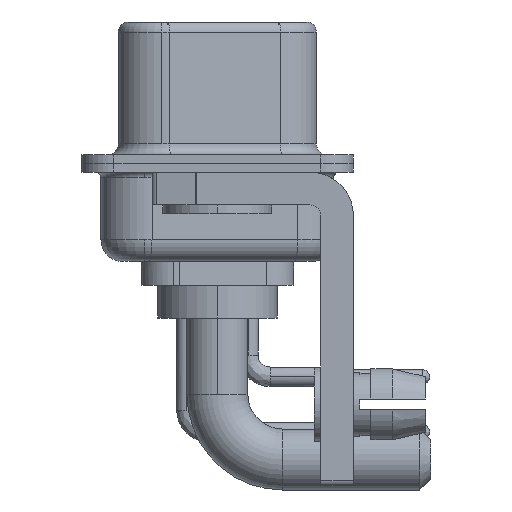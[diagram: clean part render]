
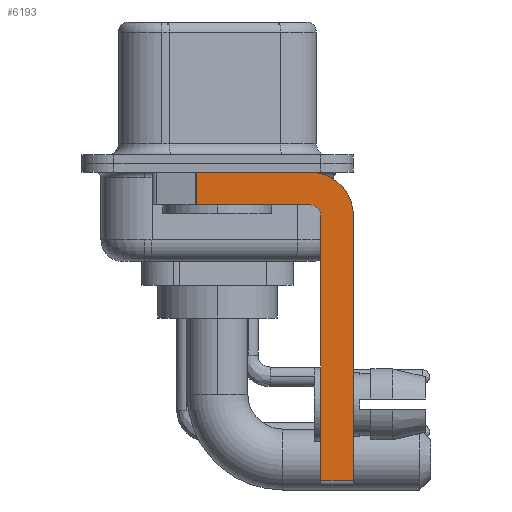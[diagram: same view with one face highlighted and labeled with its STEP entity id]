
A CAD part, left-side view. The second image highlights one B-rep face of the part: STEP entity #6193.
In plain terms, the highlighted planar face has unit normal (-1, 0, 0).
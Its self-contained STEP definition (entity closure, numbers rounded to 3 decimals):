
#279 = ORIENTED_EDGE ( 'NONE', *, *, #3281, .T. ) ;
#308 = ORIENTED_EDGE ( 'NONE', *, *, #6613, .T. ) ;
#580 = VERTEX_POINT ( 'NONE', #21489 ) ;
#977 = DIRECTION ( 'NONE',  ( 0., -1., 0. ) ) ;
#2614 = VERTEX_POINT ( 'NONE', #24230 ) ;
#2747 = VERTEX_POINT ( 'NONE', #26788 ) ;
#2781 = VERTEX_POINT ( 'NONE', #24901 ) ;
#2884 = CARTESIAN_POINT ( 'NONE',  ( -2.9, -4.25, -14.55 ) ) ;
#3281 = EDGE_CURVE ( 'NONE', #2747, #580, #25531, .T. ) ;
#3581 = EDGE_LOOP ( 'NONE', ( #22573, #279, #25792, #25350, #11338, #308, #6812, #4042 ) ) ;
#4042 = ORIENTED_EDGE ( 'NONE', *, *, #8808, .F. ) ;
#4413 = VERTEX_POINT ( 'NONE', #24467 ) ;
#4415 = VERTEX_POINT ( 'NONE', #5698 ) ;
#4446 = CARTESIAN_POINT ( 'NONE',  ( -2.9, -6.25, -2.4 ) ) ;
#4888 = DIRECTION ( 'NONE',  ( 0., 0., -1. ) ) ;
#5067 = VECTOR ( 'NONE', #977, 1000. ) ;
#5698 = CARTESIAN_POINT ( 'NONE',  ( -2.9, -4.75, -14.55 ) ) ;
#6134 = CARTESIAN_POINT ( 'NONE',  ( -2.9, -4.25, -2.4 ) ) ;
#6193 = ADVANCED_FACE ( 'NONE', ( #21496 ), #15644, .F. ) ;
#6613 = EDGE_CURVE ( 'NONE', #4415, #12518, #17320, .T. ) ;
#6812 = ORIENTED_EDGE ( 'NONE', *, *, #21670, .F. ) ;
#6926 = DIRECTION ( 'NONE',  ( 0., 0., -1. ) ) ;
#7374 = DIRECTION ( 'NONE',  ( 0., 0., -1. ) ) ;
#7470 = DIRECTION ( 'NONE',  ( 0., 0., -1. ) ) ;
#7517 = CIRCLE ( 'NONE', #9676, 0.5 ) ;
#8808 = EDGE_CURVE ( 'NONE', #4413, #26354, #25456, .T. ) ;
#8908 = LINE ( 'NONE', #9443, #19947 ) ;
#9243 = EDGE_CURVE ( 'NONE', #2747, #4413, #21679, .T. ) ;
#9312 = AXIS2_PLACEMENT_3D ( 'NONE', #11714, #11445, #4888 ) ;
#9443 = CARTESIAN_POINT ( 'NONE',  ( -2.9, -4.75, -14.8 ) ) ;
#9655 = DIRECTION ( 'NONE',  ( 0., 1., 0. ) ) ;
#9676 = AXIS2_PLACEMENT_3D ( 'NONE', #6134, #18091, #24222 ) ;
#10890 = VECTOR ( 'NONE', #7374, 1000. ) ;
#11122 = CARTESIAN_POINT ( 'NONE',  ( -2.9, 0.978, -1.9 ) ) ;
#11203 = DIRECTION ( 'NONE',  ( 0., -1., 0. ) ) ;
#11338 = ORIENTED_EDGE ( 'NONE', *, *, #20989, .F. ) ;
#11414 = CARTESIAN_POINT ( 'NONE',  ( -2.9, -4.25, -2.4 ) ) ;
#11445 = DIRECTION ( 'NONE',  ( 1., 0., 0. ) ) ;
#11714 = CARTESIAN_POINT ( 'NONE',  ( -2.9, -4.25, -2.4 ) ) ;
#11848 = LINE ( 'NONE', #24344, #10890 ) ;
#12518 = VERTEX_POINT ( 'NONE', #17530 ) ;
#13582 = DIRECTION ( 'NONE',  ( 1., 0., 0. ) ) ;
#13995 = LINE ( 'NONE', #25945, #18720 ) ;
#15644 = PLANE ( 'NONE',  #9312 ) ;
#17320 = LINE ( 'NONE', #2884, #21898 ) ;
#17530 = CARTESIAN_POINT ( 'NONE',  ( -2.9, -6.25, -14.55 ) ) ;
#18091 = DIRECTION ( 'NONE',  ( -1., 0., 0. ) ) ;
#18523 = AXIS2_PLACEMENT_3D ( 'NONE', #11414, #13582, #7470 ) ;
#18720 = VECTOR ( 'NONE', #9655, 1000. ) ;
#19947 = VECTOR ( 'NONE', #25476, 1000. ) ;
#20989 = EDGE_CURVE ( 'NONE', #4415, #2781, #8908, .T. ) ;
#21196 = VECTOR ( 'NONE', #6926, 1000. ) ;
#21489 = CARTESIAN_POINT ( 'NONE',  ( -2.9, 0.978, -1.9 ) ) ;
#21496 = FACE_OUTER_BOUND ( 'NONE', #3581, .T. ) ;
#21670 = EDGE_CURVE ( 'NONE', #26354, #12518, #11848, .T. ) ;
#21679 = LINE ( 'NONE', #26002, #5067 ) ;
#21898 = VECTOR ( 'NONE', #11203, 1000. ) ;
#22573 = ORIENTED_EDGE ( 'NONE', *, *, #9243, .F. ) ;
#24222 = DIRECTION ( 'NONE',  ( 0., 0., 1. ) ) ;
#24230 = CARTESIAN_POINT ( 'NONE',  ( -2.9, -4.25, -1.9 ) ) ;
#24344 = CARTESIAN_POINT ( 'NONE',  ( -2.9, -6.25, -2.4 ) ) ;
#24358 = EDGE_CURVE ( 'NONE', #2614, #580, #13995, .T. ) ;
#24467 = CARTESIAN_POINT ( 'NONE',  ( -2.9, -4.25, -0.4 ) ) ;
#24901 = CARTESIAN_POINT ( 'NONE',  ( -2.9, -4.75, -2.4 ) ) ;
#25350 = ORIENTED_EDGE ( 'NONE', *, *, #25757, .F. ) ;
#25456 = CIRCLE ( 'NONE', #18523, 2. ) ;
#25476 = DIRECTION ( 'NONE',  ( 0., 0., 1. ) ) ;
#25531 = LINE ( 'NONE', #11122, #21196 ) ;
#25757 = EDGE_CURVE ( 'NONE', #2781, #2614, #7517, .T. ) ;
#25792 = ORIENTED_EDGE ( 'NONE', *, *, #24358, .F. ) ;
#25945 = CARTESIAN_POINT ( 'NONE',  ( -2.9, -4.25, -1.9 ) ) ;
#26002 = CARTESIAN_POINT ( 'NONE',  ( -2.9, 3., -0.4 ) ) ;
#26354 = VERTEX_POINT ( 'NONE', #4446 ) ;
#26788 = CARTESIAN_POINT ( 'NONE',  ( -2.9, 0.978, -0.4 ) ) ;
